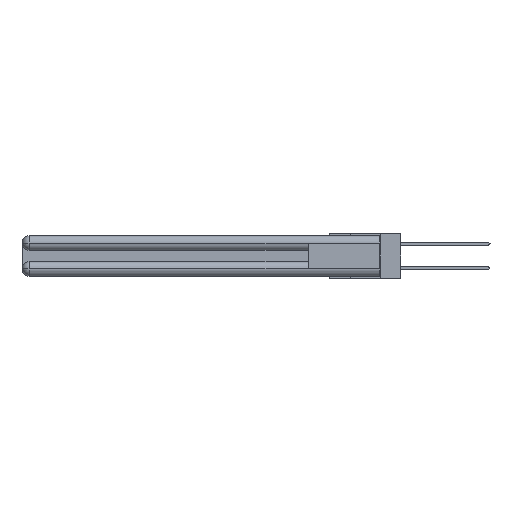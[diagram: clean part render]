
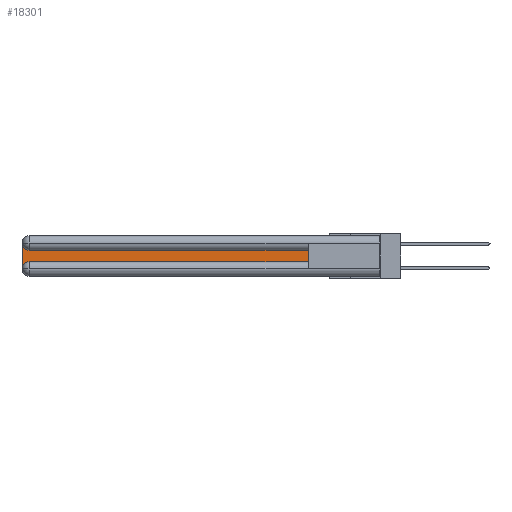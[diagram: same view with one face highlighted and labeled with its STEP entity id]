
A CAD part, left-side view. The second image highlights one B-rep face of the part: STEP entity #18301.
In plain terms, the highlighted planar face has unit normal (-1, 0, 0).
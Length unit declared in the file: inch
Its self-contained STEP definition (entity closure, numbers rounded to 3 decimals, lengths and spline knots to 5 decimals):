
#365 = DIRECTION ( 'NONE',  ( 0., 0., -1. ) ) ;
#698 = VERTEX_POINT ( 'NONE', #7272 ) ;
#1011 = ORIENTED_EDGE ( 'NONE', *, *, #28228, .T. ) ;
#1211 = FACE_OUTER_BOUND ( 'NONE', #32732, .T. ) ;
#2787 = LINE ( 'NONE', #15211, #3608 ) ;
#3608 = VECTOR ( 'NONE', #25195, 39.37008 ) ;
#4299 = VECTOR ( 'NONE', #23088, 39.37008 ) ;
#4787 = LINE ( 'NONE', #18228, #18662 ) ;
#5521 = CARTESIAN_POINT ( 'NONE',  ( 0.075, 3., -0.2175 ) ) ;
#6339 = DIRECTION ( 'NONE',  ( 0., 0., -1. ) ) ;
#7272 = CARTESIAN_POINT ( 'NONE',  ( 0.075, 0.6, -0.2175 ) ) ;
#9275 = AXIS2_PLACEMENT_3D ( 'NONE', #11474, #28737, #6339 ) ;
#10656 = EDGE_CURVE ( 'NONE', #10971, #20482, #24989, .T. ) ;
#10971 = VERTEX_POINT ( 'NONE', #27569 ) ;
#11474 = CARTESIAN_POINT ( 'NONE',  ( 0.075, 3., -0.1225 ) ) ;
#11526 = CARTESIAN_POINT ( 'NONE',  ( 0.075, 2.94, -0.0625 ) ) ;
#12082 = AXIS2_PLACEMENT_3D ( 'NONE', #11526, #29227, #16623 ) ;
#13777 = ORIENTED_EDGE ( 'NONE', *, *, #19836, .T. ) ;
#13798 = PLANE ( 'NONE',  #9275 ) ;
#13831 = AXIS2_PLACEMENT_3D ( 'NONE', #18195, #20846, #365 ) ;
#15211 = CARTESIAN_POINT ( 'NONE',  ( 0.075, 0.6, -0.2175 ) ) ;
#16614 = LINE ( 'NONE', #30762, #27694 ) ;
#16623 = DIRECTION ( 'NONE',  ( 0., 0., -1. ) ) ;
#17340 = VERTEX_POINT ( 'NONE', #28529 ) ;
#17356 = CIRCLE ( 'NONE', #12082, 0.06 ) ;
#17430 = CARTESIAN_POINT ( 'NONE',  ( 0.075, 3., -0.0625 ) ) ;
#17489 = CARTESIAN_POINT ( 'NONE',  ( 0.075, 2.94, -0.2175 ) ) ;
#18020 = EDGE_CURVE ( 'NONE', #22016, #17340, #4787, .T. ) ;
#18195 = CARTESIAN_POINT ( 'NONE',  ( 0.075, 2.94, -0.2775 ) ) ;
#18228 = CARTESIAN_POINT ( 'NONE',  ( 0.075, 0.6, -0.1225 ) ) ;
#18301 = ADVANCED_FACE ( 'NONE', ( #1211 ), #13798, .F. ) ;
#18662 = VECTOR ( 'NONE', #20776, 39.37008 ) ;
#19777 = ORIENTED_EDGE ( 'NONE', *, *, #25796, .T. ) ;
#19836 = EDGE_CURVE ( 'NONE', #20482, #698, #2787, .T. ) ;
#20148 = EDGE_CURVE ( 'NONE', #17340, #28547, #17356, .T. ) ;
#20404 = CARTESIAN_POINT ( 'NONE',  ( 0.075, 0.6, -0.1225 ) ) ;
#20482 = VERTEX_POINT ( 'NONE', #17489 ) ;
#20776 = DIRECTION ( 'NONE',  ( 0., 1., 0. ) ) ;
#20846 = DIRECTION ( 'NONE',  ( 1., 0., 0. ) ) ;
#21045 = ORIENTED_EDGE ( 'NONE', *, *, #20148, .T. ) ;
#22016 = VERTEX_POINT ( 'NONE', #20404 ) ;
#22615 = ORIENTED_EDGE ( 'NONE', *, *, #10656, .T. ) ;
#23088 = DIRECTION ( 'NONE',  ( 0., 0., -1. ) ) ;
#24086 = ORIENTED_EDGE ( 'NONE', *, *, #18020, .T. ) ;
#24989 = CIRCLE ( 'NONE', #13831, 0.06 ) ;
#25195 = DIRECTION ( 'NONE',  ( 0., -1., 0. ) ) ;
#25796 = EDGE_CURVE ( 'NONE', #698, #22016, #16614, .T. ) ;
#27569 = CARTESIAN_POINT ( 'NONE',  ( 0.075, 3., -0.2775 ) ) ;
#27694 = VECTOR ( 'NONE', #28224, 39.37008 ) ;
#28224 = DIRECTION ( 'NONE',  ( 0., 0., 1. ) ) ;
#28228 = EDGE_CURVE ( 'NONE', #28547, #10971, #28486, .T. ) ;
#28486 = LINE ( 'NONE', #5521, #4299 ) ;
#28529 = CARTESIAN_POINT ( 'NONE',  ( 0.075, 2.94, -0.1225 ) ) ;
#28547 = VERTEX_POINT ( 'NONE', #17430 ) ;
#28737 = DIRECTION ( 'NONE',  ( 1., 0., 0. ) ) ;
#29227 = DIRECTION ( 'NONE',  ( 1., 0., 0. ) ) ;
#30762 = CARTESIAN_POINT ( 'NONE',  ( 0.075, 0.6, -0.2175 ) ) ;
#32732 = EDGE_LOOP ( 'NONE', ( #24086, #21045, #1011, #22615, #13777, #19777 ) ) ;
